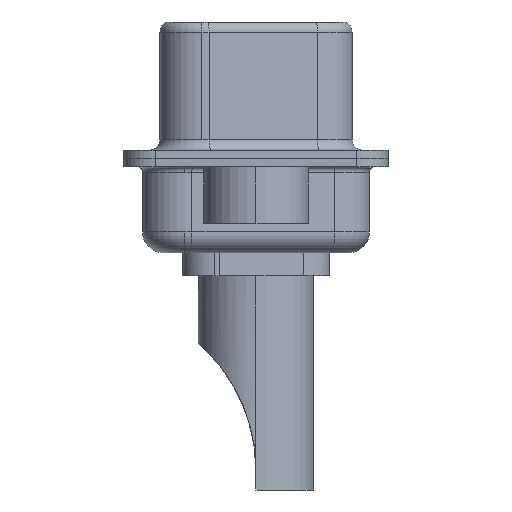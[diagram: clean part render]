
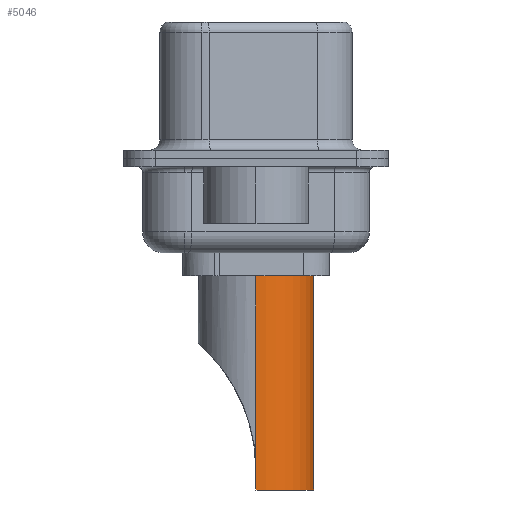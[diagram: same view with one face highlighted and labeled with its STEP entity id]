
A CAD part, left-side view. The second image highlights one B-rep face of the part: STEP entity #5046.
In plain terms, the highlighted cylindrical face has radius 2.75 mm (diameter 5.5 mm), a partial arc.
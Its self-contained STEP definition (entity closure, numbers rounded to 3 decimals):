
#10 = VERTEX_POINT ( 'NONE', #12541 ) ;
#13 = EDGE_CURVE ( 'NONE', #7588, #10, #13612, .T. ) ;
#178 = AXIS2_PLACEMENT_3D ( 'NONE', #7863, #14478, #14117 ) ;
#327 = DIRECTION ( 'NONE',  ( 0., 0., 1. ) ) ;
#358 = CARTESIAN_POINT ( 'NONE',  ( 0., 0., 4.234 ) ) ;
#533 = DIRECTION ( 'NONE',  ( 1., 0., 0. ) ) ;
#760 = VECTOR ( 'NONE', #11496, 1000. ) ;
#1068 = CARTESIAN_POINT ( 'NONE',  ( -2.75, 0., 4.234 ) ) ;
#1868 = AXIS2_PLACEMENT_3D ( 'NONE', #12719, #5232, #13891 ) ;
#2014 = CARTESIAN_POINT ( 'NONE',  ( -2.75, 0., -7.764 ) ) ;
#2409 = ORIENTED_EDGE ( 'NONE', *, *, #10928, .F. ) ;
#2482 = CARTESIAN_POINT ( 'NONE',  ( -2.75, 0., -8.7 ) ) ;
#2519 = CARTESIAN_POINT ( 'NONE',  ( 2.75, 0., 4.234 ) ) ;
#2538 = EDGE_CURVE ( 'NONE', #8646, #10, #4115, .T. ) ;
#3233 = VERTEX_POINT ( 'NONE', #8894 ) ;
#3758 = CARTESIAN_POINT ( 'NONE',  ( 2.75, 0., -7.764 ) ) ;
#4115 = CIRCLE ( 'NONE', #178, 2.75 ) ;
#4588 = ORIENTED_EDGE ( 'NONE', *, *, #9243, .T. ) ;
#4642 = VERTEX_POINT ( 'NONE', #10022 ) ;
#5046 = ADVANCED_FACE ( 'NONE', ( #10344 ), #13184, .T. ) ;
#5232 = DIRECTION ( 'NONE',  ( 0., 0., 1. ) ) ;
#6456 = VECTOR ( 'NONE', #8587, 1000. ) ;
#6532 = DIRECTION ( 'NONE',  ( 0., 0., -1. ) ) ;
#6733 = EDGE_CURVE ( 'NONE', #10724, #8646, #8555, .T. ) ;
#7539 = CIRCLE ( 'NONE', #1868, 2.75 ) ;
#7588 = VERTEX_POINT ( 'NONE', #3758 ) ;
#7863 = CARTESIAN_POINT ( 'NONE',  ( 0., 0., -8.7 ) ) ;
#8166 = VECTOR ( 'NONE', #6532, 1000. ) ;
#8555 = LINE ( 'NONE', #13887, #8166 ) ;
#8587 = DIRECTION ( 'NONE',  ( 0., 0., 1. ) ) ;
#8646 = VERTEX_POINT ( 'NONE', #2482 ) ;
#8894 = CARTESIAN_POINT ( 'NONE',  ( 2.75, 0., 1.5 ) ) ;
#9243 = EDGE_CURVE ( 'NONE', #7588, #3233, #12712, .T. ) ;
#9668 = AXIS2_PLACEMENT_3D ( 'NONE', #358, #327, #533 ) ;
#9899 = ORIENTED_EDGE ( 'NONE', *, *, #6733, .T. ) ;
#10022 = CARTESIAN_POINT ( 'NONE',  ( -2.75, 0., 1.5 ) ) ;
#10026 = DIRECTION ( 'NONE',  ( 0., 0., 1. ) ) ;
#10344 = FACE_OUTER_BOUND ( 'NONE', #14323, .T. ) ;
#10724 = VERTEX_POINT ( 'NONE', #2014 ) ;
#10928 = EDGE_CURVE ( 'NONE', #10724, #4642, #13399, .T. ) ;
#11474 = ORIENTED_EDGE ( 'NONE', *, *, #2538, .T. ) ;
#11496 = DIRECTION ( 'NONE',  ( 0., 0., -1. ) ) ;
#11519 = CARTESIAN_POINT ( 'NONE',  ( 2.75, 0., -8.7 ) ) ;
#11570 = ORIENTED_EDGE ( 'NONE', *, *, #13, .F. ) ;
#12541 = CARTESIAN_POINT ( 'NONE',  ( 2.75, 0., -8.7 ) ) ;
#12712 = LINE ( 'NONE', #2519, #15397 ) ;
#12719 = CARTESIAN_POINT ( 'NONE',  ( 0., 0., 1.5 ) ) ;
#13184 = CYLINDRICAL_SURFACE ( 'NONE', #9668, 2.75 ) ;
#13399 = LINE ( 'NONE', #1068, #6456 ) ;
#13612 = LINE ( 'NONE', #11519, #760 ) ;
#13652 = EDGE_CURVE ( 'NONE', #4642, #3233, #7539, .T. ) ;
#13887 = CARTESIAN_POINT ( 'NONE',  ( -2.75, 0., -8.7 ) ) ;
#13891 = DIRECTION ( 'NONE',  ( 1., 0., 0. ) ) ;
#13940 = ORIENTED_EDGE ( 'NONE', *, *, #13652, .F. ) ;
#14117 = DIRECTION ( 'NONE',  ( 1., 0., 0. ) ) ;
#14323 = EDGE_LOOP ( 'NONE', ( #2409, #9899, #11474, #11570, #4588, #13940 ) ) ;
#14478 = DIRECTION ( 'NONE',  ( 0., 0., 1. ) ) ;
#15397 = VECTOR ( 'NONE', #10026, 1000. ) ;
